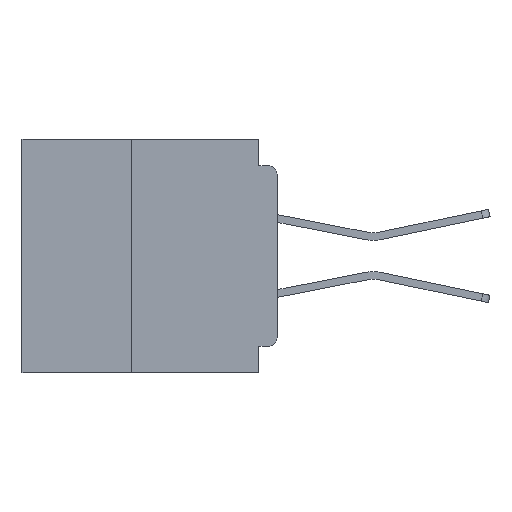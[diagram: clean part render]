
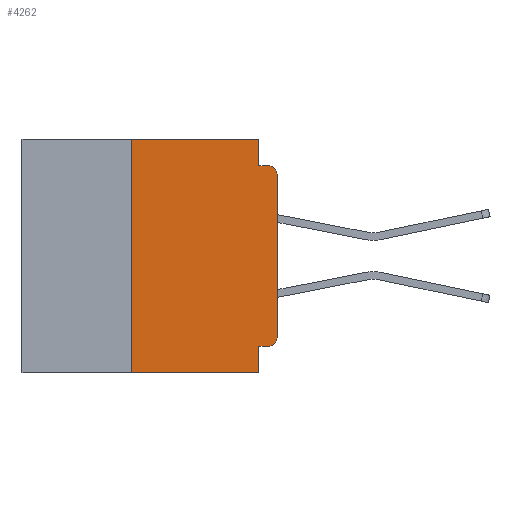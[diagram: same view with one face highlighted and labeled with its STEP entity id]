
A CAD part, left-side view. The second image highlights one B-rep face of the part: STEP entity #4262.
In plain terms, the highlighted planar face has unit normal (-1, 0, 0).
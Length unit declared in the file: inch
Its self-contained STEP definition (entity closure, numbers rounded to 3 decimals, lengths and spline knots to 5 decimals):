
#43 = VERTEX_POINT ( 'NONE', #10407 ) ;
#253 = CARTESIAN_POINT ( 'NONE',  ( 0., 0.031, -0.4 ) ) ;
#618 = VECTOR ( 'NONE', #24970, 39.37008 ) ;
#658 = ORIENTED_EDGE ( 'NONE', *, *, #2517, .F. ) ;
#1513 = AXIS2_PLACEMENT_3D ( 'NONE', #13420, #4283, #16461 ) ;
#2496 = EDGE_CURVE ( 'NONE', #6984, #17354, #35539, .T. ) ;
#2517 = EDGE_CURVE ( 'NONE', #28374, #36390, #9555, .T. ) ;
#2681 = CARTESIAN_POINT ( 'NONE',  ( 0., 0., -0.06 ) ) ;
#2761 = VERTEX_POINT ( 'NONE', #2881 ) ;
#2881 = CARTESIAN_POINT ( 'NONE',  ( 0., 0.25, -0.4 ) ) ;
#2884 = CARTESIAN_POINT ( 'NONE',  ( 0., 0., -0.34 ) ) ;
#4262 = ADVANCED_FACE ( 'NONE', ( #35387 ), #31493, .F. ) ;
#4283 = DIRECTION ( 'NONE',  ( 1., 0., 0. ) ) ;
#4585 = VECTOR ( 'NONE', #24956, 39.37008 ) ;
#6204 = CARTESIAN_POINT ( 'NONE',  ( 0., 0., -0.355 ) ) ;
#6340 = EDGE_CURVE ( 'NONE', #38501, #43, #24464, .T. ) ;
#6706 = VECTOR ( 'NONE', #15086, 39.37008 ) ;
#6984 = VERTEX_POINT ( 'NONE', #29126 ) ;
#7336 = DIRECTION ( 'NONE',  ( 0., 0., -1. ) ) ;
#7344 = DIRECTION ( 'NONE',  ( -1., 0., 0. ) ) ;
#7568 = CARTESIAN_POINT ( 'NONE',  ( 0., 0.015, -0.34 ) ) ;
#7730 = LINE ( 'NONE', #23179, #20984 ) ;
#8064 = CARTESIAN_POINT ( 'NONE',  ( 0., 0., -0.045 ) ) ;
#8108 = DIRECTION ( 'NONE',  ( 0., -1., 0. ) ) ;
#8142 = CARTESIAN_POINT ( 'NONE',  ( 0., 0.437, 0. ) ) ;
#8401 = VERTEX_POINT ( 'NONE', #253 ) ;
#8624 = LINE ( 'NONE', #27073, #6706 ) ;
#9272 = DIRECTION ( 'NONE',  ( 0., 1., 0. ) ) ;
#9555 = LINE ( 'NONE', #8142, #33637 ) ;
#9772 = CARTESIAN_POINT ( 'NONE',  ( 0., 0.031, -0.4 ) ) ;
#10301 = VECTOR ( 'NONE', #29176, 39.37008 ) ;
#10407 = CARTESIAN_POINT ( 'NONE',  ( 0., 0.015, -0.045 ) ) ;
#10905 = LINE ( 'NONE', #29568, #26967 ) ;
#11356 = DIRECTION ( 'NONE',  ( -1., 0., 0. ) ) ;
#11509 = DIRECTION ( 'NONE',  ( 0., 0., 1. ) ) ;
#11892 = CIRCLE ( 'NONE', #23977, 0.015 ) ;
#12060 = VECTOR ( 'NONE', #9272, 39.37008 ) ;
#13410 = EDGE_LOOP ( 'NONE', ( #22555, #19768, #30037, #30682, #658, #29781, #24381, #25335, #29146, #15669 ) ) ;
#13420 = CARTESIAN_POINT ( 'NONE',  ( 0., 0.437, 0. ) ) ;
#15086 = DIRECTION ( 'NONE',  ( 0., -1., 0. ) ) ;
#15539 = EDGE_CURVE ( 'NONE', #36293, #8401, #16712, .T. ) ;
#15669 = ORIENTED_EDGE ( 'NONE', *, *, #2496, .T. ) ;
#16461 = DIRECTION ( 'NONE',  ( 0., 0., -1. ) ) ;
#16712 = LINE ( 'NONE', #9772, #618 ) ;
#17354 = VERTEX_POINT ( 'NONE', #2884 ) ;
#18582 = EDGE_CURVE ( 'NONE', #20716, #43, #11892, .T. ) ;
#18975 = CARTESIAN_POINT ( 'NONE',  ( 0., 0.031, -0.045 ) ) ;
#19768 = ORIENTED_EDGE ( 'NONE', *, *, #18582, .T. ) ;
#20716 = VERTEX_POINT ( 'NONE', #2681 ) ;
#20984 = VECTOR ( 'NONE', #32277, 39.37008 ) ;
#22555 = ORIENTED_EDGE ( 'NONE', *, *, #31888, .T. ) ;
#23179 = CARTESIAN_POINT ( 'NONE',  ( 0., 0.031, 0. ) ) ;
#23798 = EDGE_CURVE ( 'NONE', #6984, #36293, #28085, .T. ) ;
#23977 = AXIS2_PLACEMENT_3D ( 'NONE', #29417, #11356, #32454 ) ;
#24381 = ORIENTED_EDGE ( 'NONE', *, *, #37708, .T. ) ;
#24464 = LINE ( 'NONE', #8064, #10301 ) ;
#24956 = DIRECTION ( 'NONE',  ( 0., 0., 1. ) ) ;
#24970 = DIRECTION ( 'NONE',  ( 0., 0., -1. ) ) ;
#25335 = ORIENTED_EDGE ( 'NONE', *, *, #15539, .F. ) ;
#26060 = EDGE_CURVE ( 'NONE', #2761, #28374, #10905, .T. ) ;
#26967 = VECTOR ( 'NONE', #11509, 39.37008 ) ;
#27073 = CARTESIAN_POINT ( 'NONE',  ( 0., 0.437, -0.4 ) ) ;
#28085 = LINE ( 'NONE', #6204, #12060 ) ;
#28112 = CARTESIAN_POINT ( 'NONE',  ( 0., 0.25, 0. ) ) ;
#28374 = VERTEX_POINT ( 'NONE', #28112 ) ;
#29062 = AXIS2_PLACEMENT_3D ( 'NONE', #7568, #7344, #7336 ) ;
#29126 = CARTESIAN_POINT ( 'NONE',  ( 0., 0.015, -0.355 ) ) ;
#29146 = ORIENTED_EDGE ( 'NONE', *, *, #23798, .F. ) ;
#29176 = DIRECTION ( 'NONE',  ( 0., -1., 0. ) ) ;
#29417 = CARTESIAN_POINT ( 'NONE',  ( 0., 0.015, -0.06 ) ) ;
#29568 = CARTESIAN_POINT ( 'NONE',  ( 0., 0.25, -0.4 ) ) ;
#29658 = LINE ( 'NONE', #30757, #4585 ) ;
#29781 = ORIENTED_EDGE ( 'NONE', *, *, #26060, .F. ) ;
#29944 = CARTESIAN_POINT ( 'NONE',  ( 0., 0.031, -0.355 ) ) ;
#30037 = ORIENTED_EDGE ( 'NONE', *, *, #6340, .F. ) ;
#30327 = CARTESIAN_POINT ( 'NONE',  ( 0., 0.031, 0. ) ) ;
#30682 = ORIENTED_EDGE ( 'NONE', *, *, #36836, .F. ) ;
#30757 = CARTESIAN_POINT ( 'NONE',  ( 0., 0., 0. ) ) ;
#31493 = PLANE ( 'NONE',  #1513 ) ;
#31888 = EDGE_CURVE ( 'NONE', #17354, #20716, #29658, .T. ) ;
#32277 = DIRECTION ( 'NONE',  ( 0., 0., -1. ) ) ;
#32454 = DIRECTION ( 'NONE',  ( 0., 0., -1. ) ) ;
#33637 = VECTOR ( 'NONE', #8108, 39.37008 ) ;
#35387 = FACE_OUTER_BOUND ( 'NONE', #13410, .T. ) ;
#35539 = CIRCLE ( 'NONE', #29062, 0.015 ) ;
#36293 = VERTEX_POINT ( 'NONE', #29944 ) ;
#36390 = VERTEX_POINT ( 'NONE', #30327 ) ;
#36836 = EDGE_CURVE ( 'NONE', #36390, #38501, #7730, .T. ) ;
#37708 = EDGE_CURVE ( 'NONE', #2761, #8401, #8624, .T. ) ;
#38501 = VERTEX_POINT ( 'NONE', #18975 ) ;
